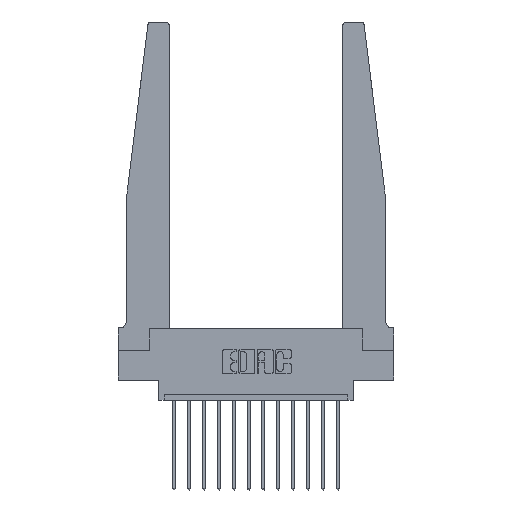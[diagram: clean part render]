
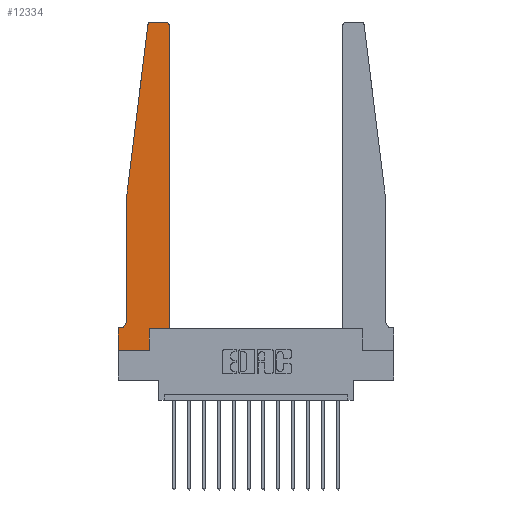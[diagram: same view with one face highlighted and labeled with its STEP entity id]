
A CAD part, top view. The second image highlights one B-rep face of the part: STEP entity #12334.
In plain terms, the highlighted planar face has unit normal (0, 0, 1).
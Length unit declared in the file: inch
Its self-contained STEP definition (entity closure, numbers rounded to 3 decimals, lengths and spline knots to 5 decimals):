
#368 = VERTEX_POINT ( 'NONE', #3693 ) ;
#752 = EDGE_CURVE ( 'NONE', #368, #3772, #9657, .T. ) ;
#904 = EDGE_CURVE ( 'NONE', #7675, #5530, #9857, .T. ) ;
#1029 = DIRECTION ( 'NONE',  ( -1., 0., 0. ) ) ;
#1123 = LINE ( 'NONE', #12864, #7363 ) ;
#1272 = CARTESIAN_POINT ( 'NONE',  ( 0.065, 0.1875, 0.37 ) ) ;
#2004 = DIRECTION ( 'NONE',  ( 0., -1., 0. ) ) ;
#2085 = CARTESIAN_POINT ( 'NONE',  ( 0.015, 0.2375, 0.37 ) ) ;
#2122 = LINE ( 'NONE', #4828, #13151 ) ;
#2205 = DIRECTION ( 'NONE',  ( 0., 1., 0. ) ) ;
#2227 = CARTESIAN_POINT ( 'NONE',  ( 0.015, 0.1875, 0.37 ) ) ;
#2378 = EDGE_CURVE ( 'NONE', #3128, #368, #8490, .T. ) ;
#2398 = VERTEX_POINT ( 'NONE', #4555 ) ;
#2444 = ORIENTED_EDGE ( 'NONE', *, *, #6998, .T. ) ;
#2565 = LINE ( 'NONE', #11272, #10046 ) ;
#2572 = DIRECTION ( 'NONE',  ( 0., 0., 1. ) ) ;
#3074 = ORIENTED_EDGE ( 'NONE', *, *, #16794, .T. ) ;
#3128 = VERTEX_POINT ( 'NONE', #3825 ) ;
#3524 = CARTESIAN_POINT ( 'NONE',  ( 0., 0., 0.37 ) ) ;
#3693 = CARTESIAN_POINT ( 'NONE',  ( 0.2605, 0.18, 0.37 ) ) ;
#3718 = CARTESIAN_POINT ( 'NONE',  ( 0.27653, 2.75, 0.37 ) ) ;
#3772 = VERTEX_POINT ( 'NONE', #14103 ) ;
#3825 = CARTESIAN_POINT ( 'NONE',  ( 0.2605, 0., 0.37 ) ) ;
#3876 = VECTOR ( 'NONE', #13664, 39.37008 ) ;
#3928 = DIRECTION ( 'NONE',  ( -1., 0., 0. ) ) ;
#3959 = CARTESIAN_POINT ( 'NONE',  ( 0.395, 2.75, 0.37 ) ) ;
#3967 = CARTESIAN_POINT ( 'NONE',  ( 0., 0.1875, 0.37 ) ) ;
#3968 = ORIENTED_EDGE ( 'NONE', *, *, #14260, .T. ) ;
#4124 = VECTOR ( 'NONE', #3928, 39.37008 ) ;
#4309 = ORIENTED_EDGE ( 'NONE', *, *, #8676, .T. ) ;
#4522 = VERTEX_POINT ( 'NONE', #2227 ) ;
#4555 = CARTESIAN_POINT ( 'NONE',  ( 0.065, 0.2375, 0.37 ) ) ;
#4787 = CARTESIAN_POINT ( 'NONE',  ( 0.065, 1.25, 0.37 ) ) ;
#4810 = VECTOR ( 'NONE', #7204, 39.37008 ) ;
#4828 = CARTESIAN_POINT ( 'NONE',  ( 0.425, 0.18, 0.37 ) ) ;
#4859 = ORIENTED_EDGE ( 'NONE', *, *, #904, .T. ) ;
#4884 = AXIS2_PLACEMENT_3D ( 'NONE', #16772, #9032, #15429 ) ;
#4968 = ORIENTED_EDGE ( 'NONE', *, *, #2378, .T. ) ;
#5281 = AXIS2_PLACEMENT_3D ( 'NONE', #2085, #9741, #7271 ) ;
#5304 = ORIENTED_EDGE ( 'NONE', *, *, #7381, .T. ) ;
#5327 = DIRECTION ( 'NONE',  ( 1., 0., 0. ) ) ;
#5530 = VERTEX_POINT ( 'NONE', #7476 ) ;
#6374 = DIRECTION ( 'NONE',  ( 0., 0., 1. ) ) ;
#6445 = PLANE ( 'NONE',  #9316 ) ;
#6483 = LINE ( 'NONE', #11937, #4124 ) ;
#6744 = ORIENTED_EDGE ( 'NONE', *, *, #752, .T. ) ;
#6893 = VERTEX_POINT ( 'NONE', #14867 ) ;
#6998 = EDGE_CURVE ( 'NONE', #7017, #14951, #12781, .T. ) ;
#7017 = VERTEX_POINT ( 'NONE', #7457 ) ;
#7204 = DIRECTION ( 'NONE',  ( 0., 1., 0. ) ) ;
#7271 = DIRECTION ( 'NONE',  ( -1., 0., 0. ) ) ;
#7363 = VECTOR ( 'NONE', #16436, 39.37008 ) ;
#7381 = EDGE_CURVE ( 'NONE', #5530, #14832, #1123, .T. ) ;
#7457 = CARTESIAN_POINT ( 'NONE',  ( 0.425, 2.72, 0.37 ) ) ;
#7476 = CARTESIAN_POINT ( 'NONE',  ( 0.24675, 2.72367, 0.37 ) ) ;
#7602 = CARTESIAN_POINT ( 'NONE',  ( 0.27653, 2.72, 0.37 ) ) ;
#7675 = VERTEX_POINT ( 'NONE', #3718 ) ;
#7767 = DIRECTION ( 'NONE',  ( 1., 0., 0. ) ) ;
#7900 = FACE_OUTER_BOUND ( 'NONE', #8518, .T. ) ;
#8245 = VERTEX_POINT ( 'NONE', #3524 ) ;
#8490 = LINE ( 'NONE', #10952, #4810 ) ;
#8518 = EDGE_LOOP ( 'NONE', ( #11911, #4859, #5304, #12011, #11388, #3074, #3968, #4309, #4968, #6744, #15058, #2444 ) ) ;
#8676 = EDGE_CURVE ( 'NONE', #8245, #3128, #2565, .T. ) ;
#8794 = LINE ( 'NONE', #16362, #3876 ) ;
#9032 = DIRECTION ( 'NONE',  ( 0., 0., 1. ) ) ;
#9316 = AXIS2_PLACEMENT_3D ( 'NONE', #3967, #6374, #5327 ) ;
#9657 = LINE ( 'NONE', #9908, #12297 ) ;
#9741 = DIRECTION ( 'NONE',  ( 0., 0., -1. ) ) ;
#9857 = CIRCLE ( 'NONE', #12030, 0.03 ) ;
#9908 = CARTESIAN_POINT ( 'NONE',  ( 0.425, 0.18, 0.37 ) ) ;
#10046 = VECTOR ( 'NONE', #16439, 39.37008 ) ;
#10952 = CARTESIAN_POINT ( 'NONE',  ( 0.2605, 0.18, 0.37 ) ) ;
#11272 = CARTESIAN_POINT ( 'NONE',  ( 0., 0., 0.37 ) ) ;
#11388 = ORIENTED_EDGE ( 'NONE', *, *, #14364, .T. ) ;
#11467 = EDGE_CURVE ( 'NONE', #14951, #7675, #6483, .T. ) ;
#11557 = VECTOR ( 'NONE', #1029, 39.37008 ) ;
#11911 = ORIENTED_EDGE ( 'NONE', *, *, #11467, .T. ) ;
#11937 = CARTESIAN_POINT ( 'NONE',  ( 0.25, 2.75, 0.37 ) ) ;
#12011 = ORIENTED_EDGE ( 'NONE', *, *, #14275, .T. ) ;
#12030 = AXIS2_PLACEMENT_3D ( 'NONE', #7602, #2572, #7767 ) ;
#12297 = VECTOR ( 'NONE', #15269, 39.37008 ) ;
#12334 = ADVANCED_FACE ( 'NONE', ( #7900 ), #6445, .T. ) ;
#12553 = LINE ( 'NONE', #4787, #12899 ) ;
#12604 = CARTESIAN_POINT ( 'NONE',  ( 0.065, 1.25, 0.37 ) ) ;
#12781 = CIRCLE ( 'NONE', #4884, 0.03 ) ;
#12864 = CARTESIAN_POINT ( 'NONE',  ( 0.065, 1.25, 0.37 ) ) ;
#12899 = VECTOR ( 'NONE', #2004, 39.37008 ) ;
#13151 = VECTOR ( 'NONE', #2205, 39.37008 ) ;
#13462 = EDGE_CURVE ( 'NONE', #3772, #7017, #2122, .T. ) ;
#13664 = DIRECTION ( 'NONE',  ( 0., -1., 0. ) ) ;
#14043 = LINE ( 'NONE', #1272, #11557 ) ;
#14103 = CARTESIAN_POINT ( 'NONE',  ( 0.425, 0.18, 0.37 ) ) ;
#14260 = EDGE_CURVE ( 'NONE', #6893, #8245, #8794, .T. ) ;
#14275 = EDGE_CURVE ( 'NONE', #14832, #2398, #12553, .T. ) ;
#14364 = EDGE_CURVE ( 'NONE', #2398, #4522, #14538, .T. ) ;
#14538 = CIRCLE ( 'NONE', #5281, 0.05 ) ;
#14832 = VERTEX_POINT ( 'NONE', #12604 ) ;
#14867 = CARTESIAN_POINT ( 'NONE',  ( 0., 0.1875, 0.37 ) ) ;
#14951 = VERTEX_POINT ( 'NONE', #3959 ) ;
#15058 = ORIENTED_EDGE ( 'NONE', *, *, #13462, .T. ) ;
#15269 = DIRECTION ( 'NONE',  ( 1., 0., 0. ) ) ;
#15429 = DIRECTION ( 'NONE',  ( 1., 0., 0. ) ) ;
#16362 = CARTESIAN_POINT ( 'NONE',  ( 0., 0., 0.37 ) ) ;
#16436 = DIRECTION ( 'NONE',  ( -0.122, -0.992, 0. ) ) ;
#16439 = DIRECTION ( 'NONE',  ( 1., 0., 0. ) ) ;
#16772 = CARTESIAN_POINT ( 'NONE',  ( 0.395, 2.72, 0.37 ) ) ;
#16794 = EDGE_CURVE ( 'NONE', #4522, #6893, #14043, .T. ) ;
